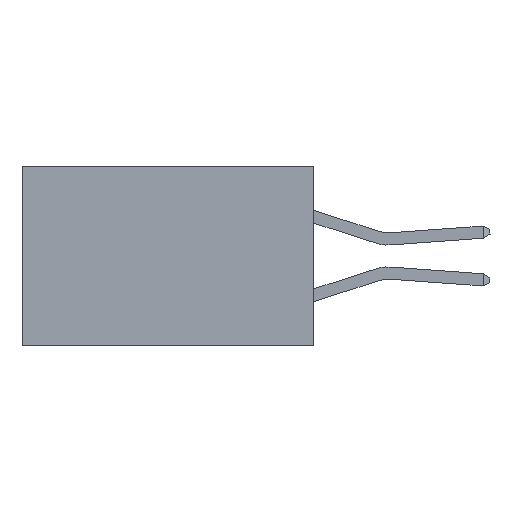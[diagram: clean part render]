
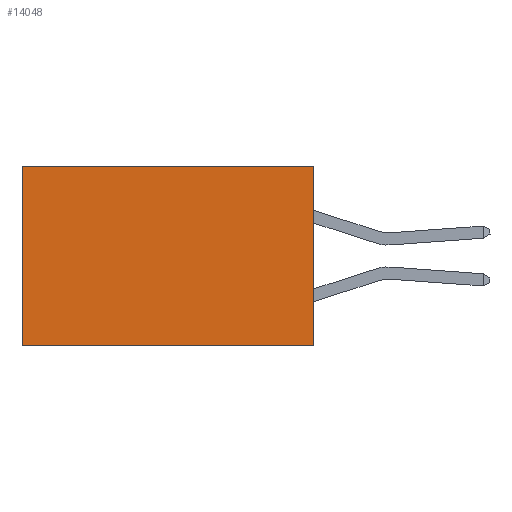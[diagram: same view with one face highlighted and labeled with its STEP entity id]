
A CAD part, left-side view. The second image highlights one B-rep face of the part: STEP entity #14048.
In plain terms, the highlighted planar face has unit normal (-1, 0, 0).
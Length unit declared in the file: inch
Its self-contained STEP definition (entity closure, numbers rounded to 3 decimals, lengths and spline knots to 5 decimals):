
#120 = EDGE_CURVE ( 'NONE', #1390, #7814, #548, .T. ) ;
#168 = CARTESIAN_POINT ( 'NONE',  ( 0.2875, 0., 0. ) ) ;
#548 = LINE ( 'NONE', #6261, #9046 ) ;
#1143 = CARTESIAN_POINT ( 'NONE',  ( 0.2875, 0., 0. ) ) ;
#1390 = VERTEX_POINT ( 'NONE', #9832 ) ;
#1439 = DIRECTION ( 'NONE',  ( 0., 0., -1. ) ) ;
#2124 = ORIENTED_EDGE ( 'NONE', *, *, #10811, .T. ) ;
#2454 = DIRECTION ( 'NONE',  ( 0., 1., 0. ) ) ;
#2687 = DIRECTION ( 'NONE',  ( 0., 0., -1. ) ) ;
#2736 = VECTOR ( 'NONE', #2687, 39.37008 ) ;
#3250 = CARTESIAN_POINT ( 'NONE',  ( 0.2875, 0., 0. ) ) ;
#3353 = CARTESIAN_POINT ( 'NONE',  ( 0.2875, 0.6, 0. ) ) ;
#3371 = EDGE_CURVE ( 'NONE', #13037, #7814, #8469, .T. ) ;
#4589 = DIRECTION ( 'NONE',  ( 0., 1., 0. ) ) ;
#4828 = EDGE_LOOP ( 'NONE', ( #6569, #13556, #12390, #2124 ) ) ;
#5420 = VECTOR ( 'NONE', #2454, 39.37008 ) ;
#6261 = CARTESIAN_POINT ( 'NONE',  ( 0.2875, 0., -0.37 ) ) ;
#6569 = ORIENTED_EDGE ( 'NONE', *, *, #3371, .T. ) ;
#6643 = CARTESIAN_POINT ( 'NONE',  ( 0.2875, 0.6, 0. ) ) ;
#6713 = CARTESIAN_POINT ( 'NONE',  ( 0.2875, 0.6, -0.37 ) ) ;
#7236 = PLANE ( 'NONE',  #10854 ) ;
#7814 = VERTEX_POINT ( 'NONE', #6713 ) ;
#8133 = VECTOR ( 'NONE', #11304, 39.37008 ) ;
#8363 = DIRECTION ( 'NONE',  ( 1., 0., 0. ) ) ;
#8469 = LINE ( 'NONE', #3353, #2736 ) ;
#8504 = EDGE_CURVE ( 'NONE', #10055, #1390, #11345, .T. ) ;
#9046 = VECTOR ( 'NONE', #4589, 39.37008 ) ;
#9832 = CARTESIAN_POINT ( 'NONE',  ( 0.2875, 0., -0.37 ) ) ;
#10055 = VERTEX_POINT ( 'NONE', #3250 ) ;
#10220 = CARTESIAN_POINT ( 'NONE',  ( 0.2875, 0., 0. ) ) ;
#10378 = FACE_OUTER_BOUND ( 'NONE', #4828, .T. ) ;
#10811 = EDGE_CURVE ( 'NONE', #10055, #13037, #10988, .T. ) ;
#10854 = AXIS2_PLACEMENT_3D ( 'NONE', #168, #8363, #1439 ) ;
#10988 = LINE ( 'NONE', #1143, #5420 ) ;
#11304 = DIRECTION ( 'NONE',  ( 0., 0., -1. ) ) ;
#11345 = LINE ( 'NONE', #10220, #8133 ) ;
#12390 = ORIENTED_EDGE ( 'NONE', *, *, #8504, .F. ) ;
#13037 = VERTEX_POINT ( 'NONE', #6643 ) ;
#13556 = ORIENTED_EDGE ( 'NONE', *, *, #120, .F. ) ;
#14048 = ADVANCED_FACE ( 'NONE', ( #10378 ), #7236, .F. ) ;
